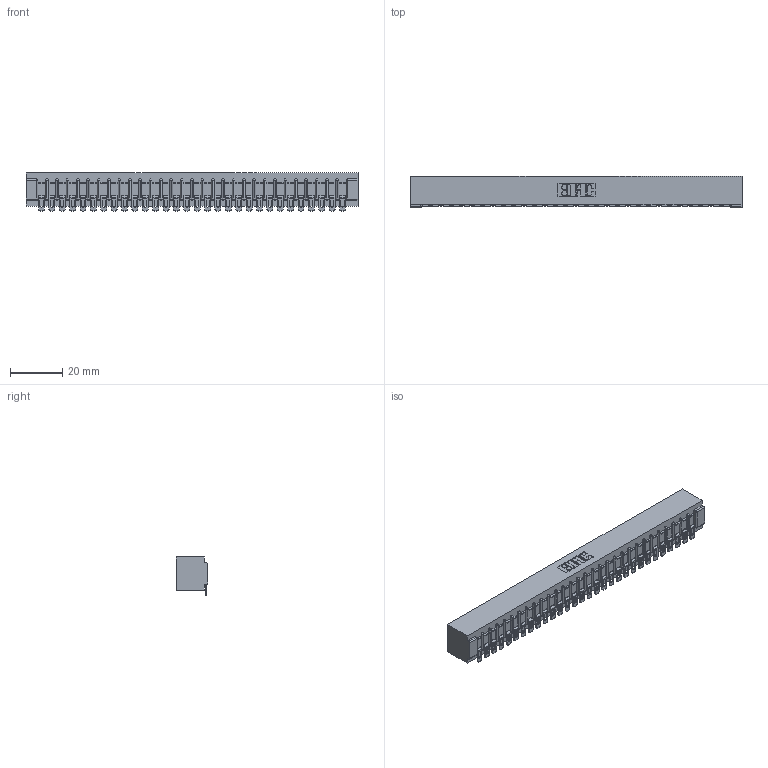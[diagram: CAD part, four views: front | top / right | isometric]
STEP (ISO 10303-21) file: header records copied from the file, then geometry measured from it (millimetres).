
FILE_DESCRIPTION (( 'STEP AP203' ), '1' );
FILE_NAME ('307-030-554-101.STEP', '2019-09-05T04:22:03', ( '' ), ( '' ), 'SwSTEP 2.0', 'SolidWorks 2016', '' );
FILE_SCHEMA (( 'CONFIG_CONTROL_DESIGN' ));
Length unit declared in the file: inch
Products named in the file (3): 307-290-002_554; 307 Part_No Mounting Lugs; 307-030-554-101
Assembly tree (31 placements, depth 2):
  307-030-554-101
    307 Part_No Mounting Lugs
    307-290-002_554  x30
Bounding box: 126.75 x 12.01 x 14.52 mm (x, y, z)
Volume: 14042.5 mm3; surface area: 17859 mm2
Topology: 31 solids, 31 shells, 2571 faces, 7889 edges, 5174 vertices
Faces by surface type: plane 1446, cylinder 1063, sphere 62
Entity records: 27885 total; most frequent: CARTESIAN_POINT 4702, ORIENTED_EDGE 4692, DIRECTION 4578, EDGE_CURVE 2346, VECTOR 1786, LINE 1786, VERTEX_POINT 1520, AXIS2_PLACEMENT_3D 1396
